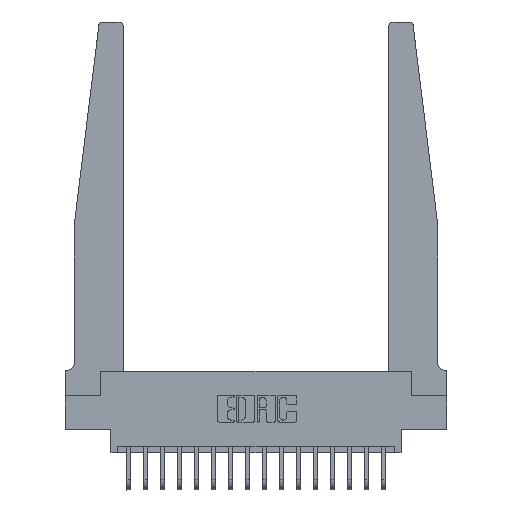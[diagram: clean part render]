
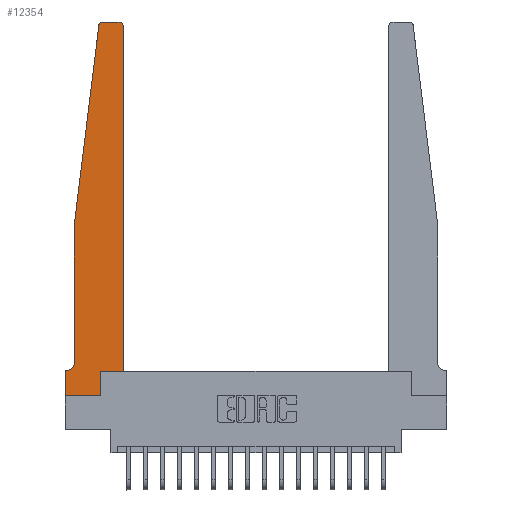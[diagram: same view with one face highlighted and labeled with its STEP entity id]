
A CAD part, top view. The second image highlights one B-rep face of the part: STEP entity #12354.
In plain terms, the highlighted planar face has unit normal (0, 0, 1).
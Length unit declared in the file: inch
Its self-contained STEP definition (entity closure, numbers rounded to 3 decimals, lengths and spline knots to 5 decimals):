
#205 = EDGE_CURVE ( 'NONE', #4348, #4203, #18759, .T. ) ;
#245 = DIRECTION ( 'NONE',  ( 0., 0., 1. ) ) ;
#701 = EDGE_CURVE ( 'NONE', #17695, #10166, #11003, .T. ) ;
#717 = EDGE_CURVE ( 'NONE', #10554, #17695, #6293, .T. ) ;
#983 = CARTESIAN_POINT ( 'NONE',  ( 0.065, 1.25, 0.37 ) ) ;
#1180 = CARTESIAN_POINT ( 'NONE',  ( 0., 0., 0.37 ) ) ;
#1407 = EDGE_CURVE ( 'NONE', #16273, #4461, #19867, .T. ) ;
#1461 = VECTOR ( 'NONE', #7089, 39.37008 ) ;
#1720 = EDGE_LOOP ( 'NONE', ( #16522, #20018, #19954, #6678, #17919, #8828, #9481, #4564, #3712, #17953, #10739, #14158 ) ) ;
#1856 = PLANE ( 'NONE',  #8552 ) ;
#2613 = CARTESIAN_POINT ( 'NONE',  ( 0.015, 0.1875, 0.37 ) ) ;
#2679 = CARTESIAN_POINT ( 'NONE',  ( 0., 0.1875, 0.37 ) ) ;
#3114 = EDGE_CURVE ( 'NONE', #3595, #19059, #10685, .T. ) ;
#3406 = CIRCLE ( 'NONE', #18946, 0.03 ) ;
#3595 = VERTEX_POINT ( 'NONE', #20166 ) ;
#3712 = ORIENTED_EDGE ( 'NONE', *, *, #8314, .T. ) ;
#3828 = CARTESIAN_POINT ( 'NONE',  ( 0.425, 2.72, 0.37 ) ) ;
#3895 = DIRECTION ( 'NONE',  ( -1., 0., 0. ) ) ;
#4203 = VERTEX_POINT ( 'NONE', #2613 ) ;
#4348 = VERTEX_POINT ( 'NONE', #12107 ) ;
#4461 = VERTEX_POINT ( 'NONE', #3828 ) ;
#4564 = ORIENTED_EDGE ( 'NONE', *, *, #701, .T. ) ;
#5437 = EDGE_CURVE ( 'NONE', #4461, #12701, #11333, .T. ) ;
#5442 = CARTESIAN_POINT ( 'NONE',  ( 0.065, 0.1875, 0.37 ) ) ;
#5483 = VERTEX_POINT ( 'NONE', #12796 ) ;
#5621 = DIRECTION ( 'NONE',  ( 0., -1., 0. ) ) ;
#6293 = LINE ( 'NONE', #20256, #13583 ) ;
#6336 = EDGE_CURVE ( 'NONE', #4203, #10554, #7064, .T. ) ;
#6603 = VECTOR ( 'NONE', #8385, 39.37008 ) ;
#6676 = DIRECTION ( 'NONE',  ( 1., 0., 0. ) ) ;
#6678 = ORIENTED_EDGE ( 'NONE', *, *, #8340, .T. ) ;
#7064 = LINE ( 'NONE', #5442, #16290 ) ;
#7089 = DIRECTION ( 'NONE',  ( 0., 1., 0. ) ) ;
#7194 = VECTOR ( 'NONE', #9500, 39.37008 ) ;
#7576 = VECTOR ( 'NONE', #11822, 39.37008 ) ;
#7698 = CARTESIAN_POINT ( 'NONE',  ( 0.395, 2.72, 0.37 ) ) ;
#8117 = LINE ( 'NONE', #983, #20518 ) ;
#8314 = EDGE_CURVE ( 'NONE', #10166, #5483, #15228, .T. ) ;
#8340 = EDGE_CURVE ( 'NONE', #19059, #4348, #8117, .T. ) ;
#8385 = DIRECTION ( 'NONE',  ( -1., 0., 0. ) ) ;
#8452 = FACE_OUTER_BOUND ( 'NONE', #1720, .T. ) ;
#8552 = AXIS2_PLACEMENT_3D ( 'NONE', #9813, #16095, #6676 ) ;
#8828 = ORIENTED_EDGE ( 'NONE', *, *, #6336, .T. ) ;
#8981 = EDGE_CURVE ( 'NONE', #5483, #16273, #16281, .T. ) ;
#9158 = DIRECTION ( 'NONE',  ( 1., 0., 0. ) ) ;
#9297 = CARTESIAN_POINT ( 'NONE',  ( 0.065, 1.25, 0.37 ) ) ;
#9481 = ORIENTED_EDGE ( 'NONE', *, *, #717, .T. ) ;
#9500 = DIRECTION ( 'NONE',  ( -0.122, -0.992, 0. ) ) ;
#9813 = CARTESIAN_POINT ( 'NONE',  ( 0., 0.1875, 0.37 ) ) ;
#10166 = VERTEX_POINT ( 'NONE', #12721 ) ;
#10330 = LINE ( 'NONE', #14747, #6603 ) ;
#10554 = VERTEX_POINT ( 'NONE', #2679 ) ;
#10685 = LINE ( 'NONE', #9297, #7194 ) ;
#10739 = ORIENTED_EDGE ( 'NONE', *, *, #1407, .T. ) ;
#10894 = DIRECTION ( 'NONE',  ( 1., 0., 0. ) ) ;
#11003 = LINE ( 'NONE', #13835, #14763 ) ;
#11154 = DIRECTION ( 'NONE',  ( 1., 0., 0. ) ) ;
#11333 = CIRCLE ( 'NONE', #17911, 0.03 ) ;
#11822 = DIRECTION ( 'NONE',  ( 1., 0., 0. ) ) ;
#12107 = CARTESIAN_POINT ( 'NONE',  ( 0.065, 0.2375, 0.37 ) ) ;
#12158 = AXIS2_PLACEMENT_3D ( 'NONE', #13590, #12249, #13857 ) ;
#12249 = DIRECTION ( 'NONE',  ( 0., 0., -1. ) ) ;
#12354 = ADVANCED_FACE ( 'NONE', ( #8452 ), #1856, .T. ) ;
#12688 = CARTESIAN_POINT ( 'NONE',  ( 0.425, 0.18, 0.37 ) ) ;
#12701 = VERTEX_POINT ( 'NONE', #18056 ) ;
#12721 = CARTESIAN_POINT ( 'NONE',  ( 0.2605, 0., 0.37 ) ) ;
#12796 = CARTESIAN_POINT ( 'NONE',  ( 0.2605, 0.18, 0.37 ) ) ;
#13583 = VECTOR ( 'NONE', #16995, 39.37008 ) ;
#13590 = CARTESIAN_POINT ( 'NONE',  ( 0.015, 0.2375, 0.37 ) ) ;
#13835 = CARTESIAN_POINT ( 'NONE',  ( 0., 0., 0.37 ) ) ;
#13857 = DIRECTION ( 'NONE',  ( -1., 0., 0. ) ) ;
#13871 = EDGE_CURVE ( 'NONE', #18122, #3595, #3406, .T. ) ;
#14118 = DIRECTION ( 'NONE',  ( 0., 0., 1. ) ) ;
#14158 = ORIENTED_EDGE ( 'NONE', *, *, #5437, .T. ) ;
#14747 = CARTESIAN_POINT ( 'NONE',  ( 0.25, 2.75, 0.37 ) ) ;
#14763 = VECTOR ( 'NONE', #9158, 39.37008 ) ;
#15024 = CARTESIAN_POINT ( 'NONE',  ( 0.2605, 0.18, 0.37 ) ) ;
#15228 = LINE ( 'NONE', #15024, #1461 ) ;
#15250 = EDGE_CURVE ( 'NONE', #12701, #18122, #10330, .T. ) ;
#15789 = CARTESIAN_POINT ( 'NONE',  ( 0.065, 1.25, 0.37 ) ) ;
#16095 = DIRECTION ( 'NONE',  ( 0., 0., 1. ) ) ;
#16273 = VERTEX_POINT ( 'NONE', #12688 ) ;
#16281 = LINE ( 'NONE', #17997, #7576 ) ;
#16290 = VECTOR ( 'NONE', #3895, 39.37008 ) ;
#16447 = CARTESIAN_POINT ( 'NONE',  ( 0.27653, 2.75, 0.37 ) ) ;
#16522 = ORIENTED_EDGE ( 'NONE', *, *, #15250, .T. ) ;
#16995 = DIRECTION ( 'NONE',  ( 0., -1., 0. ) ) ;
#17615 = VECTOR ( 'NONE', #19147, 39.37008 ) ;
#17682 = CARTESIAN_POINT ( 'NONE',  ( 0.27653, 2.72, 0.37 ) ) ;
#17695 = VERTEX_POINT ( 'NONE', #1180 ) ;
#17911 = AXIS2_PLACEMENT_3D ( 'NONE', #7698, #14118, #10894 ) ;
#17919 = ORIENTED_EDGE ( 'NONE', *, *, #205, .T. ) ;
#17953 = ORIENTED_EDGE ( 'NONE', *, *, #8981, .T. ) ;
#17997 = CARTESIAN_POINT ( 'NONE',  ( 0.425, 0.18, 0.37 ) ) ;
#18056 = CARTESIAN_POINT ( 'NONE',  ( 0.395, 2.75, 0.37 ) ) ;
#18122 = VERTEX_POINT ( 'NONE', #16447 ) ;
#18759 = CIRCLE ( 'NONE', #12158, 0.05 ) ;
#18946 = AXIS2_PLACEMENT_3D ( 'NONE', #17682, #245, #11154 ) ;
#19059 = VERTEX_POINT ( 'NONE', #15789 ) ;
#19147 = DIRECTION ( 'NONE',  ( 0., 1., 0. ) ) ;
#19286 = CARTESIAN_POINT ( 'NONE',  ( 0.425, 0.18, 0.37 ) ) ;
#19867 = LINE ( 'NONE', #19286, #17615 ) ;
#19954 = ORIENTED_EDGE ( 'NONE', *, *, #3114, .T. ) ;
#20018 = ORIENTED_EDGE ( 'NONE', *, *, #13871, .T. ) ;
#20166 = CARTESIAN_POINT ( 'NONE',  ( 0.24675, 2.72367, 0.37 ) ) ;
#20256 = CARTESIAN_POINT ( 'NONE',  ( 0., 0., 0.37 ) ) ;
#20518 = VECTOR ( 'NONE', #5621, 39.37008 ) ;
